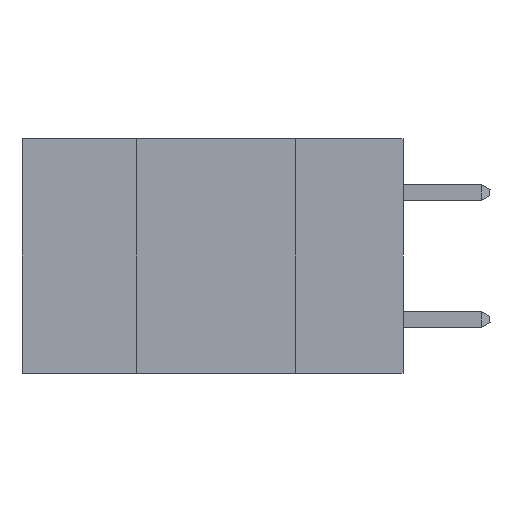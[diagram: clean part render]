
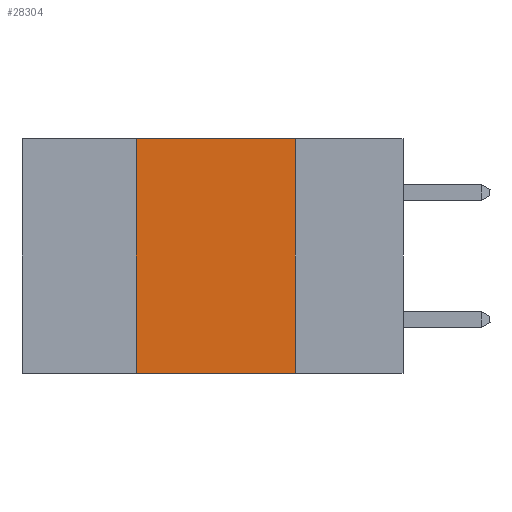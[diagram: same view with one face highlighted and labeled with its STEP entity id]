
A CAD part, left-side view. The second image highlights one B-rep face of the part: STEP entity #28304.
In plain terms, the highlighted planar face has unit normal (-1, 0, 0).
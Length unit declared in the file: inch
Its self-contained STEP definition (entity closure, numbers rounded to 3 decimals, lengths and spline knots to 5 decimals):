
#1342 = EDGE_CURVE ( 'NONE', #5445, #12502, #33921, .T. ) ;
#2549 = DIRECTION ( 'NONE',  ( 0., -1., 0. ) ) ;
#3728 = DIRECTION ( 'NONE',  ( 0., 0., 1. ) ) ;
#4775 = EDGE_CURVE ( 'NONE', #37231, #12502, #33714, .T. ) ;
#5281 = VERTEX_POINT ( 'NONE', #40129 ) ;
#5445 = VERTEX_POINT ( 'NONE', #5717 ) ;
#5717 = CARTESIAN_POINT ( 'NONE',  ( 0., 0.17, 0. ) ) ;
#12502 = VERTEX_POINT ( 'NONE', #42691 ) ;
#12836 = VECTOR ( 'NONE', #3728, 39.37008 ) ;
#15489 = ORIENTED_EDGE ( 'NONE', *, *, #29134, .F. ) ;
#15648 = CARTESIAN_POINT ( 'NONE',  ( 0., 0.6, -0.37 ) ) ;
#15744 = ORIENTED_EDGE ( 'NONE', *, *, #29379, .F. ) ;
#16136 = LINE ( 'NONE', #41250, #43022 ) ;
#17188 = LINE ( 'NONE', #21429, #12836 ) ;
#17911 = DIRECTION ( 'NONE',  ( 1., 0., 0. ) ) ;
#21429 = CARTESIAN_POINT ( 'NONE',  ( 0., 0.42, 0. ) ) ;
#21490 = ORIENTED_EDGE ( 'NONE', *, *, #4775, .T. ) ;
#23519 = VECTOR ( 'NONE', #34837, 39.37008 ) ;
#24978 = VECTOR ( 'NONE', #26543, 39.37008 ) ;
#25139 = CARTESIAN_POINT ( 'NONE',  ( 0., 0.6, 0. ) ) ;
#26543 = DIRECTION ( 'NONE',  ( 0., -1., 0. ) ) ;
#28304 = ADVANCED_FACE ( 'NONE', ( #29900 ), #35370, .F. ) ;
#28354 = DIRECTION ( 'NONE',  ( 0., 0., -1. ) ) ;
#29134 = EDGE_CURVE ( 'NONE', #5281, #5445, #16136, .T. ) ;
#29379 = EDGE_CURVE ( 'NONE', #37231, #5281, #17188, .T. ) ;
#29900 = FACE_OUTER_BOUND ( 'NONE', #32612, .T. ) ;
#30040 = CARTESIAN_POINT ( 'NONE',  ( 0., 0.17, 0. ) ) ;
#32612 = EDGE_LOOP ( 'NONE', ( #44363, #15489, #15744, #21490 ) ) ;
#33714 = LINE ( 'NONE', #15648, #24978 ) ;
#33921 = LINE ( 'NONE', #30040, #23519 ) ;
#34837 = DIRECTION ( 'NONE',  ( 0., 0., -1. ) ) ;
#35370 = PLANE ( 'NONE',  #43099 ) ;
#37231 = VERTEX_POINT ( 'NONE', #37402 ) ;
#37402 = CARTESIAN_POINT ( 'NONE',  ( 0., 0.42, -0.37 ) ) ;
#40129 = CARTESIAN_POINT ( 'NONE',  ( 0., 0.42, 0. ) ) ;
#41250 = CARTESIAN_POINT ( 'NONE',  ( 0., 0.6, 0. ) ) ;
#42691 = CARTESIAN_POINT ( 'NONE',  ( 0., 0.17, -0.37 ) ) ;
#43022 = VECTOR ( 'NONE', #2549, 39.37008 ) ;
#43099 = AXIS2_PLACEMENT_3D ( 'NONE', #25139, #17911, #28354 ) ;
#44363 = ORIENTED_EDGE ( 'NONE', *, *, #1342, .F. ) ;
